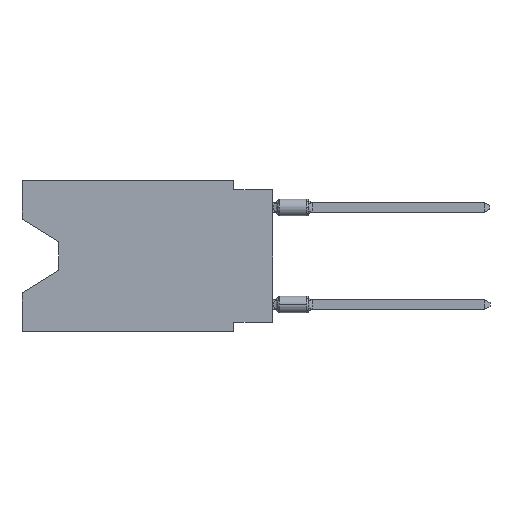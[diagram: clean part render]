
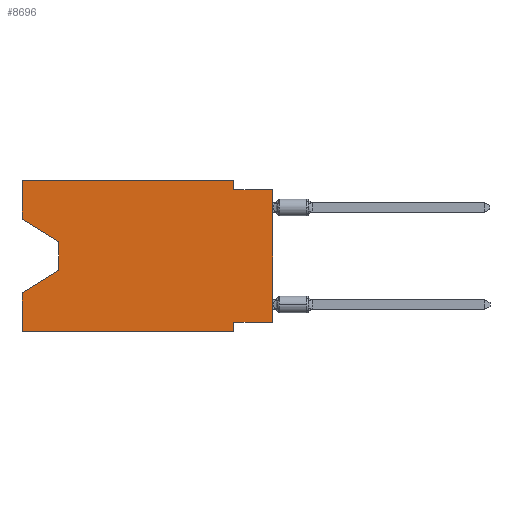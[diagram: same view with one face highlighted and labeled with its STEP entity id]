
A CAD part, left-side view. The second image highlights one B-rep face of the part: STEP entity #8696.
In plain terms, the highlighted planar face has unit normal (-1, 0, 0).
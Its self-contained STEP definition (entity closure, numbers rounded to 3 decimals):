
#224 = DIRECTION ( 'NONE',  ( 0., 0., -1. ) ) ;
#241 = DIRECTION ( 'NONE',  ( 0., 1., 0. ) ) ;
#312 = VECTOR ( 'NONE', #4317, 1000. ) ;
#393 = DIRECTION ( 'NONE',  ( 0., 0.855, -0.519 ) ) ;
#548 = DIRECTION ( 'NONE',  ( 0., 0., 1. ) ) ;
#781 = CARTESIAN_POINT ( 'NONE',  ( 0., 2.54, -9.906 ) ) ;
#842 = EDGE_CURVE ( 'NONE', #6364, #9166, #7551, .T. ) ;
#1079 = CARTESIAN_POINT ( 'NONE',  ( 0., 13.97, -4.013 ) ) ;
#1231 = LINE ( 'NONE', #5229, #11847 ) ;
#1336 = CARTESIAN_POINT ( 'NONE',  ( 0., 16.383, 0. ) ) ;
#1531 = VERTEX_POINT ( 'NONE', #10537 ) ;
#1805 = CARTESIAN_POINT ( 'NONE',  ( 0., 2.54, -9.906 ) ) ;
#1826 = LINE ( 'NONE', #781, #11391 ) ;
#2066 = FACE_OUTER_BOUND ( 'NONE', #3796, .T. ) ;
#2251 = ORIENTED_EDGE ( 'NONE', *, *, #6514, .F. ) ;
#2287 = VERTEX_POINT ( 'NONE', #9189 ) ;
#2321 = VECTOR ( 'NONE', #2382, 1000. ) ;
#2335 = DIRECTION ( 'NONE',  ( 0., 0., 1. ) ) ;
#2382 = DIRECTION ( 'NONE',  ( 0., -1., 0. ) ) ;
#2506 = CARTESIAN_POINT ( 'NONE',  ( 0., 16.383, -9.906 ) ) ;
#2645 = VECTOR ( 'NONE', #9143, 1000. ) ;
#2800 = LINE ( 'NONE', #3854, #4216 ) ;
#2822 = AXIS2_PLACEMENT_3D ( 'NONE', #7193, #10208, #224 ) ;
#2835 = VECTOR ( 'NONE', #393, 1000. ) ;
#3010 = VERTEX_POINT ( 'NONE', #12897 ) ;
#3131 = LINE ( 'NONE', #8129, #5993 ) ;
#3166 = ORIENTED_EDGE ( 'NONE', *, *, #9221, .T. ) ;
#3189 = PLANE ( 'NONE',  #2822 ) ;
#3319 = LINE ( 'NONE', #1336, #2321 ) ;
#3542 = ORIENTED_EDGE ( 'NONE', *, *, #3942, .F. ) ;
#3695 = ORIENTED_EDGE ( 'NONE', *, *, #7836, .T. ) ;
#3796 = EDGE_LOOP ( 'NONE', ( #3695, #3901, #3166, #3542, #6081, #12702, #2251, #5695, #5798, #4470, #5898, #5723 ) ) ;
#3854 = CARTESIAN_POINT ( 'NONE',  ( 0., 16.383, 0. ) ) ;
#3887 = VERTEX_POINT ( 'NONE', #5966 ) ;
#3901 = ORIENTED_EDGE ( 'NONE', *, *, #5774, .T. ) ;
#3942 = EDGE_CURVE ( 'NONE', #5848, #6823, #3131, .T. ) ;
#4121 = LINE ( 'NONE', #10086, #312 ) ;
#4212 = VERTEX_POINT ( 'NONE', #1805 ) ;
#4216 = VECTOR ( 'NONE', #7865, 1000. ) ;
#4317 = DIRECTION ( 'NONE',  ( 0., 0., -1. ) ) ;
#4470 = ORIENTED_EDGE ( 'NONE', *, *, #6445, .F. ) ;
#5011 = DIRECTION ( 'NONE',  ( 0., 0., -1. ) ) ;
#5144 = VERTEX_POINT ( 'NONE', #10956 ) ;
#5229 = CARTESIAN_POINT ( 'NONE',  ( 0., 0., -9.271 ) ) ;
#5331 = VERTEX_POINT ( 'NONE', #11213 ) ;
#5455 = CARTESIAN_POINT ( 'NONE',  ( 0., 13.97, -5.893 ) ) ;
#5541 = CARTESIAN_POINT ( 'NONE',  ( 0., 0., 0. ) ) ;
#5588 = DIRECTION ( 'NONE',  ( 0., -1., 0. ) ) ;
#5695 = ORIENTED_EDGE ( 'NONE', *, *, #8839, .T. ) ;
#5723 = ORIENTED_EDGE ( 'NONE', *, *, #9800, .F. ) ;
#5774 = EDGE_CURVE ( 'NONE', #3887, #1531, #6994, .T. ) ;
#5798 = ORIENTED_EDGE ( 'NONE', *, *, #842, .F. ) ;
#5848 = VERTEX_POINT ( 'NONE', #2506 ) ;
#5898 = ORIENTED_EDGE ( 'NONE', *, *, #12286, .F. ) ;
#5966 = CARTESIAN_POINT ( 'NONE',  ( 0., 13.97, -4.013 ) ) ;
#5993 = VECTOR ( 'NONE', #2335, 1000. ) ;
#6081 = ORIENTED_EDGE ( 'NONE', *, *, #7301, .T. ) ;
#6364 = VERTEX_POINT ( 'NONE', #9969 ) ;
#6445 = EDGE_CURVE ( 'NONE', #3010, #6364, #4121, .T. ) ;
#6514 = EDGE_CURVE ( 'NONE', #5144, #5331, #1231, .T. ) ;
#6595 = CARTESIAN_POINT ( 'NONE',  ( 0., 16.383, -2.546 ) ) ;
#6823 = VERTEX_POINT ( 'NONE', #8045 ) ;
#6879 = DIRECTION ( 'NONE',  ( 0., 0., -1. ) ) ;
#6994 = LINE ( 'NONE', #1079, #9359 ) ;
#7043 = VERTEX_POINT ( 'NONE', #6595 ) ;
#7173 = LINE ( 'NONE', #11182, #2645 ) ;
#7193 = CARTESIAN_POINT ( 'NONE',  ( 0., 16.383, 0. ) ) ;
#7301 = EDGE_CURVE ( 'NONE', #5848, #4212, #7173, .T. ) ;
#7551 = LINE ( 'NONE', #11687, #12200 ) ;
#7670 = LINE ( 'NONE', #10674, #11872 ) ;
#7836 = EDGE_CURVE ( 'NONE', #7043, #3887, #7670, .T. ) ;
#7865 = DIRECTION ( 'NONE',  ( 0., 0., 1. ) ) ;
#8045 = CARTESIAN_POINT ( 'NONE',  ( 0., 16.383, -7.36 ) ) ;
#8129 = CARTESIAN_POINT ( 'NONE',  ( 0., 16.383, 0. ) ) ;
#8696 = ADVANCED_FACE ( 'NONE', ( #2066 ), #3189, .F. ) ;
#8839 = EDGE_CURVE ( 'NONE', #5144, #9166, #10533, .T. ) ;
#9143 = DIRECTION ( 'NONE',  ( 0., -1., 0. ) ) ;
#9166 = VERTEX_POINT ( 'NONE', #10194 ) ;
#9189 = CARTESIAN_POINT ( 'NONE',  ( 0., 16.383, 0. ) ) ;
#9221 = EDGE_CURVE ( 'NONE', #1531, #6823, #11376, .T. ) ;
#9328 = VECTOR ( 'NONE', #548, 1000. ) ;
#9359 = VECTOR ( 'NONE', #5011, 1000. ) ;
#9800 = EDGE_CURVE ( 'NONE', #7043, #2287, #2800, .T. ) ;
#9969 = CARTESIAN_POINT ( 'NONE',  ( 0., 2.54, -0.635 ) ) ;
#10086 = CARTESIAN_POINT ( 'NONE',  ( 0., 2.54, 0. ) ) ;
#10194 = CARTESIAN_POINT ( 'NONE',  ( 0., 0., -0.635 ) ) ;
#10208 = DIRECTION ( 'NONE',  ( 1., 0., 0. ) ) ;
#10533 = LINE ( 'NONE', #5541, #9328 ) ;
#10537 = CARTESIAN_POINT ( 'NONE',  ( 0., 13.97, -5.893 ) ) ;
#10674 = CARTESIAN_POINT ( 'NONE',  ( 0., 16.383, -2.546 ) ) ;
#10956 = CARTESIAN_POINT ( 'NONE',  ( 0., 0., -9.271 ) ) ;
#11182 = CARTESIAN_POINT ( 'NONE',  ( 0., 16.383, -9.906 ) ) ;
#11213 = CARTESIAN_POINT ( 'NONE',  ( 0., 2.54, -9.271 ) ) ;
#11376 = LINE ( 'NONE', #5455, #2835 ) ;
#11391 = VECTOR ( 'NONE', #6879, 1000. ) ;
#11648 = EDGE_CURVE ( 'NONE', #5331, #4212, #1826, .T. ) ;
#11687 = CARTESIAN_POINT ( 'NONE',  ( 0., 0., -0.635 ) ) ;
#11847 = VECTOR ( 'NONE', #241, 1000. ) ;
#11872 = VECTOR ( 'NONE', #12715, 1000. ) ;
#12200 = VECTOR ( 'NONE', #5588, 1000. ) ;
#12286 = EDGE_CURVE ( 'NONE', #2287, #3010, #3319, .T. ) ;
#12702 = ORIENTED_EDGE ( 'NONE', *, *, #11648, .F. ) ;
#12715 = DIRECTION ( 'NONE',  ( 0., -0.855, -0.519 ) ) ;
#12897 = CARTESIAN_POINT ( 'NONE',  ( 0., 2.54, 0. ) ) ;
